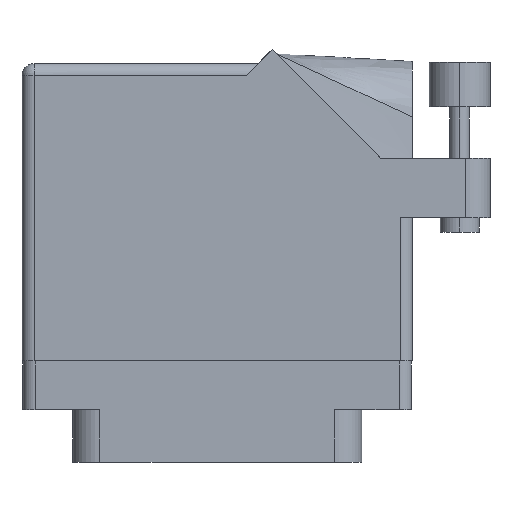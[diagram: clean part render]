
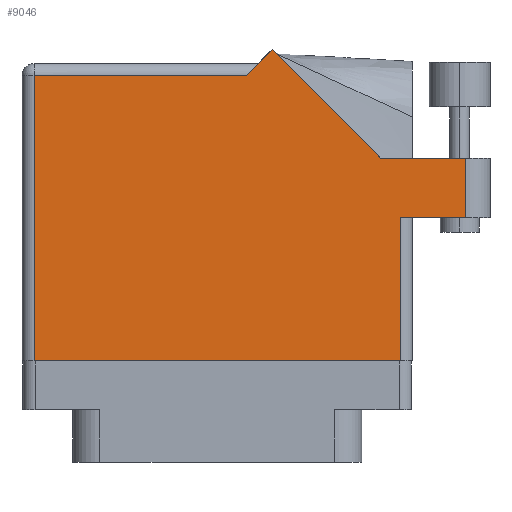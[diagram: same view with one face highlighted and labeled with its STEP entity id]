
A CAD part, front view. The second image highlights one B-rep face of the part: STEP entity #9046.
In plain terms, the highlighted face is planar.
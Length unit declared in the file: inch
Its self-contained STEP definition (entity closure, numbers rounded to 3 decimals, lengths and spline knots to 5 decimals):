
#791 = DIRECTION ( 'NONE',  ( -1., 0., 0. ) ) ;
#825 = VECTOR ( 'NONE', #35012, 39.37008 ) ;
#909 = VECTOR ( 'NONE', #8288, 39.37008 ) ;
#1245 = EDGE_CURVE ( 'NONE', #23324, #5644, #24140, .T. ) ;
#1428 = CARTESIAN_POINT ( 'NONE',  ( 1.005, 0.637, 0.455 ) ) ;
#2484 = ORIENTED_EDGE ( 'NONE', *, *, #1245, .T. ) ;
#4018 = CARTESIAN_POINT ( 'NONE',  ( 0.943, 0.637, 0.455 ) ) ;
#4932 = CARTESIAN_POINT ( 'NONE',  ( 0.943, -0.1, 0.455 ) ) ;
#5573 = CARTESIAN_POINT ( 'NONE',  ( -0.943, 1.368, 0.455 ) ) ;
#5644 = VERTEX_POINT ( 'NONE', #25267 ) ;
#6691 = VERTEX_POINT ( 'NONE', #35333 ) ;
#7289 = ORIENTED_EDGE ( 'NONE', *, *, #16960, .T. ) ;
#7639 = PLANE ( 'NONE',  #14936 ) ;
#7779 = CARTESIAN_POINT ( 'NONE',  ( -1.005, 1.43, 0.455 ) ) ;
#8218 = EDGE_CURVE ( 'NONE', #32376, #23324, #14880, .T. ) ;
#8282 = EDGE_CURVE ( 'NONE', #6691, #21754, #37635, .T. ) ;
#8288 = DIRECTION ( 'NONE',  ( -1., 0., 0. ) ) ;
#8701 = EDGE_LOOP ( 'NONE', ( #36056, #2484, #7289, #10182, #29301, #33731, #35190, #39526, #22868 ) ) ;
#9046 = ADVANCED_FACE ( 'NONE', ( #36411 ), #7639, .F. ) ;
#9118 = LINE ( 'NONE', #36046, #909 ) ;
#10182 = ORIENTED_EDGE ( 'NONE', *, *, #13429, .T. ) ;
#10460 = CARTESIAN_POINT ( 'NONE',  ( 1.28, 0.637, 0.455 ) ) ;
#10648 = LINE ( 'NONE', #17687, #32042 ) ;
#10990 = LINE ( 'NONE', #16658, #31376 ) ;
#12488 = DIRECTION ( 'NONE',  ( 0., -1., 0. ) ) ;
#13429 = EDGE_CURVE ( 'NONE', #17210, #27395, #35555, .T. ) ;
#14880 = LINE ( 'NONE', #1428, #825 ) ;
#14936 = AXIS2_PLACEMENT_3D ( 'NONE', #7779, #19464, #791 ) ;
#16658 = CARTESIAN_POINT ( 'NONE',  ( -0.943, -0.1, 0.455 ) ) ;
#16741 = CARTESIAN_POINT ( 'NONE',  ( 0.212, 1.43, 0.455 ) ) ;
#16960 = EDGE_CURVE ( 'NONE', #5644, #17210, #9118, .T. ) ;
#16984 = VERTEX_POINT ( 'NONE', #5573 ) ;
#17210 = VERTEX_POINT ( 'NONE', #31689 ) ;
#17687 = CARTESIAN_POINT ( 'NONE',  ( 0.943, 0.637, 0.455 ) ) ;
#17703 = VECTOR ( 'NONE', #28230, 39.37008 ) ;
#19392 = EDGE_CURVE ( 'NONE', #32111, #16984, #29336, .T. ) ;
#19464 = DIRECTION ( 'NONE',  ( 0., 0., -1. ) ) ;
#20430 = DIRECTION ( 'NONE',  ( 0., 1., 0. ) ) ;
#21754 = VERTEX_POINT ( 'NONE', #4932 ) ;
#22868 = ORIENTED_EDGE ( 'NONE', *, *, #28253, .T. ) ;
#23068 = VECTOR ( 'NONE', #28841, 39.37008 ) ;
#23324 = VERTEX_POINT ( 'NONE', #10460 ) ;
#23576 = EDGE_CURVE ( 'NONE', #16984, #6691, #10990, .T. ) ;
#23617 = DIRECTION ( 'NONE',  ( 1., 0., 0. ) ) ;
#23720 = DIRECTION ( 'NONE',  ( 0., 1., 0. ) ) ;
#24140 = LINE ( 'NONE', #26573, #28535 ) ;
#24470 = CARTESIAN_POINT ( 'NONE',  ( 0.28271, 1.50071, 0.455 ) ) ;
#24672 = EDGE_CURVE ( 'NONE', #27395, #32111, #38054, .T. ) ;
#25267 = CARTESIAN_POINT ( 'NONE',  ( 1.28, 0.944, 0.455 ) ) ;
#26573 = CARTESIAN_POINT ( 'NONE',  ( 1.28, 0.944, 0.455 ) ) ;
#27354 = VECTOR ( 'NONE', #37375, 39.37008 ) ;
#27395 = VERTEX_POINT ( 'NONE', #24470 ) ;
#28230 = DIRECTION ( 'NONE',  ( -1., 0., 0. ) ) ;
#28253 = EDGE_CURVE ( 'NONE', #21754, #32376, #10648, .T. ) ;
#28535 = VECTOR ( 'NONE', #23720, 39.37008 ) ;
#28841 = DIRECTION ( 'NONE',  ( -0.707, -0.707, 0. ) ) ;
#29301 = ORIENTED_EDGE ( 'NONE', *, *, #24672, .T. ) ;
#29336 = LINE ( 'NONE', #34166, #17703 ) ;
#31376 = VECTOR ( 'NONE', #12488, 39.37008 ) ;
#31689 = CARTESIAN_POINT ( 'NONE',  ( 0.83942, 0.944, 0.455 ) ) ;
#32042 = VECTOR ( 'NONE', #20430, 39.37008 ) ;
#32111 = VERTEX_POINT ( 'NONE', #36794 ) ;
#32376 = VERTEX_POINT ( 'NONE', #4018 ) ;
#32969 = CARTESIAN_POINT ( 'NONE',  ( -1.005, -0.1, 0.455 ) ) ;
#33731 = ORIENTED_EDGE ( 'NONE', *, *, #19392, .T. ) ;
#34166 = CARTESIAN_POINT ( 'NONE',  ( -1.005, 1.368, 0.455 ) ) ;
#34748 = VECTOR ( 'NONE', #23617, 39.37008 ) ;
#35012 = DIRECTION ( 'NONE',  ( 1., 0., 0. ) ) ;
#35190 = ORIENTED_EDGE ( 'NONE', *, *, #23576, .T. ) ;
#35333 = CARTESIAN_POINT ( 'NONE',  ( -0.943, -0.1, 0.455 ) ) ;
#35555 = LINE ( 'NONE', #37902, #27354 ) ;
#36046 = CARTESIAN_POINT ( 'NONE',  ( 1.405, 0.944, 0.455 ) ) ;
#36056 = ORIENTED_EDGE ( 'NONE', *, *, #8218, .T. ) ;
#36411 = FACE_OUTER_BOUND ( 'NONE', #8701, .T. ) ;
#36794 = CARTESIAN_POINT ( 'NONE',  ( 0.15, 1.368, 0.455 ) ) ;
#37375 = DIRECTION ( 'NONE',  ( -0.707, 0.707, 0. ) ) ;
#37635 = LINE ( 'NONE', #32969, #34748 ) ;
#37902 = CARTESIAN_POINT ( 'NONE',  ( 0.83942, 0.944, 0.455 ) ) ;
#38054 = LINE ( 'NONE', #16741, #23068 ) ;
#39526 = ORIENTED_EDGE ( 'NONE', *, *, #8282, .T. ) ;
